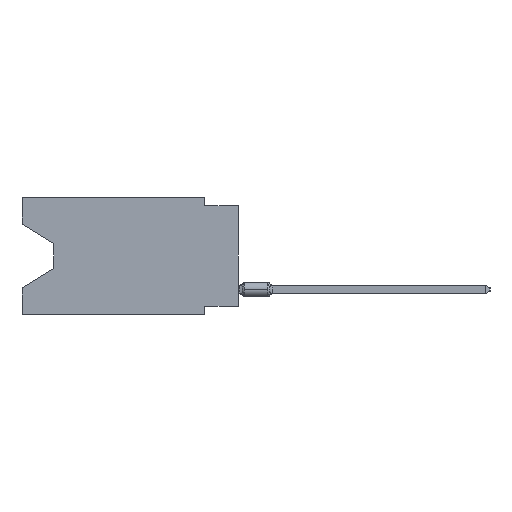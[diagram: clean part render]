
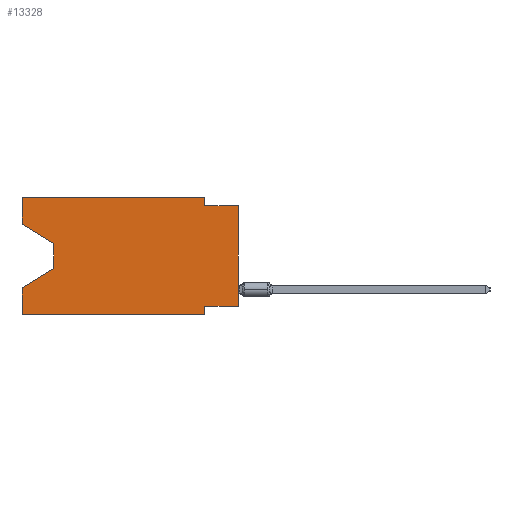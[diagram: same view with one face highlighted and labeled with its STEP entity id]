
A CAD part, left-side view. The second image highlights one B-rep face of the part: STEP entity #13328.
In plain terms, the highlighted planar face has unit normal (-1, 0, 0).
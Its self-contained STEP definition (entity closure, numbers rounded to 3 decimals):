
#365 = FACE_OUTER_BOUND ( 'NONE', #11002, .T. ) ;
#378 = ORIENTED_EDGE ( 'NONE', *, *, #42772, .T. ) ;
#687 = LINE ( 'NONE', #41693, #8934 ) ;
#708 = VERTEX_POINT ( 'NONE', #25511 ) ;
#942 = VECTOR ( 'NONE', #48496, 1000. ) ;
#1020 = VECTOR ( 'NONE', #40035, 1000. ) ;
#1024 = ORIENTED_EDGE ( 'NONE', *, *, #11206, .F. ) ;
#1071 = EDGE_CURVE ( 'NONE', #9316, #9447, #687, .T. ) ;
#1147 = EDGE_CURVE ( 'NONE', #3127, #34799, #55533, .T. ) ;
#1232 = DIRECTION ( 'NONE',  ( 0., 0., -1. ) ) ;
#2226 = ORIENTED_EDGE ( 'NONE', *, *, #16568, .F. ) ;
#2607 = ORIENTED_EDGE ( 'NONE', *, *, #31170, .T. ) ;
#2670 = VECTOR ( 'NONE', #15835, 1000. ) ;
#2716 = DIRECTION ( 'NONE',  ( 0., 0., -1. ) ) ;
#2754 = DIRECTION ( 'NONE',  ( 0., 0., -1. ) ) ;
#3127 = VERTEX_POINT ( 'NONE', #57465 ) ;
#3910 = LINE ( 'NONE', #31357, #942 ) ;
#4456 = ORIENTED_EDGE ( 'NONE', *, *, #1147, .F. ) ;
#4885 = LINE ( 'NONE', #41457, #14459 ) ;
#5959 = DIRECTION ( 'NONE',  ( 1., 0., 0. ) ) ;
#7849 = VERTEX_POINT ( 'NONE', #8427 ) ;
#8427 = CARTESIAN_POINT ( 'NONE',  ( 0., 0., -8.255 ) ) ;
#8464 = LINE ( 'NONE', #26179, #31551 ) ;
#8830 = ORIENTED_EDGE ( 'NONE', *, *, #25268, .T. ) ;
#8934 = VECTOR ( 'NONE', #28137, 1000. ) ;
#8953 = VERTEX_POINT ( 'NONE', #42978 ) ;
#9316 = VERTEX_POINT ( 'NONE', #38330 ) ;
#9447 = VERTEX_POINT ( 'NONE', #39491 ) ;
#10397 = PLANE ( 'NONE',  #38908 ) ;
#11002 = EDGE_LOOP ( 'NONE', ( #50696, #55085, #2607, #24467, #378, #56835, #39478, #8830, #1024, #4456, #2226, #49883 ) ) ;
#11206 = EDGE_CURVE ( 'NONE', #34799, #13533, #51551, .T. ) ;
#12031 = CARTESIAN_POINT ( 'NONE',  ( 0., 0., -0.635 ) ) ;
#12473 = DIRECTION ( 'NONE',  ( 0., 0., -1. ) ) ;
#13320 = VECTOR ( 'NONE', #35641, 1000. ) ;
#13328 = ADVANCED_FACE ( 'NONE', ( #365 ), #10397, .F. ) ;
#13533 = VERTEX_POINT ( 'NONE', #57273 ) ;
#14459 = VECTOR ( 'NONE', #24033, 1000. ) ;
#14874 = EDGE_CURVE ( 'NONE', #8953, #19121, #16343, .T. ) ;
#14995 = VERTEX_POINT ( 'NONE', #52913 ) ;
#15467 = CARTESIAN_POINT ( 'NONE',  ( 0., 13.97, -3.505 ) ) ;
#15835 = DIRECTION ( 'NONE',  ( 0., 1., 0. ) ) ;
#16343 = LINE ( 'NONE', #15467, #17360 ) ;
#16568 = EDGE_CURVE ( 'NONE', #9447, #3127, #39916, .T. ) ;
#16890 = CARTESIAN_POINT ( 'NONE',  ( 0., 2.54, -8.89 ) ) ;
#17360 = VECTOR ( 'NONE', #2754, 1000. ) ;
#19121 = VERTEX_POINT ( 'NONE', #22723 ) ;
#21166 = DIRECTION ( 'NONE',  ( 0., 0.855, -0.519 ) ) ;
#21533 = CARTESIAN_POINT ( 'NONE',  ( 0., 2.54, -8.89 ) ) ;
#21541 = CARTESIAN_POINT ( 'NONE',  ( 0., 16.383, -2.038 ) ) ;
#21797 = EDGE_CURVE ( 'NONE', #7849, #14995, #24087, .T. ) ;
#22354 = LINE ( 'NONE', #40926, #13320 ) ;
#22723 = CARTESIAN_POINT ( 'NONE',  ( 0., 13.97, -5.385 ) ) ;
#23097 = VECTOR ( 'NONE', #2716, 1000. ) ;
#24033 = DIRECTION ( 'NONE',  ( 0., -1., 0. ) ) ;
#24087 = LINE ( 'NONE', #42374, #2670 ) ;
#24467 = ORIENTED_EDGE ( 'NONE', *, *, #26279, .F. ) ;
#25268 = EDGE_CURVE ( 'NONE', #7849, #13533, #3910, .T. ) ;
#25511 = CARTESIAN_POINT ( 'NONE',  ( 0., 16.383, -6.852 ) ) ;
#26179 = CARTESIAN_POINT ( 'NONE',  ( 0., 13.97, -5.385 ) ) ;
#26279 = EDGE_CURVE ( 'NONE', #41824, #708, #22354, .T. ) ;
#27106 = CARTESIAN_POINT ( 'NONE',  ( 0., 2.54, -0.635 ) ) ;
#27109 = CARTESIAN_POINT ( 'NONE',  ( 0., 16.383, -8.89 ) ) ;
#28137 = DIRECTION ( 'NONE',  ( 0., 0., 1. ) ) ;
#28343 = VECTOR ( 'NONE', #12473, 1000. ) ;
#31045 = LINE ( 'NONE', #16890, #28343 ) ;
#31170 = EDGE_CURVE ( 'NONE', #19121, #708, #8464, .T. ) ;
#31357 = CARTESIAN_POINT ( 'NONE',  ( 0., 0., 0. ) ) ;
#31551 = VECTOR ( 'NONE', #21166, 1000. ) ;
#33873 = VECTOR ( 'NONE', #39239, 1000. ) ;
#34738 = VERTEX_POINT ( 'NONE', #21533 ) ;
#34799 = VERTEX_POINT ( 'NONE', #27106 ) ;
#35552 = EDGE_CURVE ( 'NONE', #14995, #34738, #31045, .T. ) ;
#35641 = DIRECTION ( 'NONE',  ( 0., 0., 1. ) ) ;
#38330 = CARTESIAN_POINT ( 'NONE',  ( 0., 16.383, -2.038 ) ) ;
#38393 = EDGE_CURVE ( 'NONE', #9316, #8953, #56935, .T. ) ;
#38908 = AXIS2_PLACEMENT_3D ( 'NONE', #41668, #5959, #1232 ) ;
#39239 = DIRECTION ( 'NONE',  ( 0., -0.855, -0.519 ) ) ;
#39478 = ORIENTED_EDGE ( 'NONE', *, *, #21797, .F. ) ;
#39491 = CARTESIAN_POINT ( 'NONE',  ( 0., 16.383, 0. ) ) ;
#39916 = LINE ( 'NONE', #44355, #47500 ) ;
#40035 = DIRECTION ( 'NONE',  ( 0., -1., 0. ) ) ;
#40926 = CARTESIAN_POINT ( 'NONE',  ( 0., 16.383, 0. ) ) ;
#41457 = CARTESIAN_POINT ( 'NONE',  ( 0., 16.383, -8.89 ) ) ;
#41668 = CARTESIAN_POINT ( 'NONE',  ( 0., 16.383, 0. ) ) ;
#41693 = CARTESIAN_POINT ( 'NONE',  ( 0., 16.383, 0. ) ) ;
#41824 = VERTEX_POINT ( 'NONE', #27109 ) ;
#42374 = CARTESIAN_POINT ( 'NONE',  ( 0., 0., -8.255 ) ) ;
#42564 = CARTESIAN_POINT ( 'NONE',  ( 0., 2.54, 0. ) ) ;
#42772 = EDGE_CURVE ( 'NONE', #41824, #34738, #4885, .T. ) ;
#42978 = CARTESIAN_POINT ( 'NONE',  ( 0., 13.97, -3.505 ) ) ;
#44066 = DIRECTION ( 'NONE',  ( 0., -1., 0. ) ) ;
#44355 = CARTESIAN_POINT ( 'NONE',  ( 0., 16.383, 0. ) ) ;
#47500 = VECTOR ( 'NONE', #44066, 1000. ) ;
#48496 = DIRECTION ( 'NONE',  ( 0., 0., 1. ) ) ;
#49883 = ORIENTED_EDGE ( 'NONE', *, *, #1071, .F. ) ;
#50696 = ORIENTED_EDGE ( 'NONE', *, *, #38393, .T. ) ;
#51551 = LINE ( 'NONE', #12031, #1020 ) ;
#52913 = CARTESIAN_POINT ( 'NONE',  ( 0., 2.54, -8.255 ) ) ;
#55085 = ORIENTED_EDGE ( 'NONE', *, *, #14874, .T. ) ;
#55533 = LINE ( 'NONE', #42564, #23097 ) ;
#56835 = ORIENTED_EDGE ( 'NONE', *, *, #35552, .F. ) ;
#56935 = LINE ( 'NONE', #21541, #33873 ) ;
#57273 = CARTESIAN_POINT ( 'NONE',  ( 0., 0., -0.635 ) ) ;
#57465 = CARTESIAN_POINT ( 'NONE',  ( 0., 2.54, 0. ) ) ;
